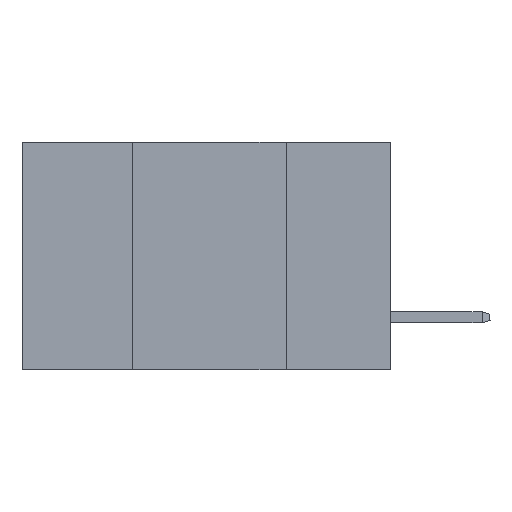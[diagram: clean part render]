
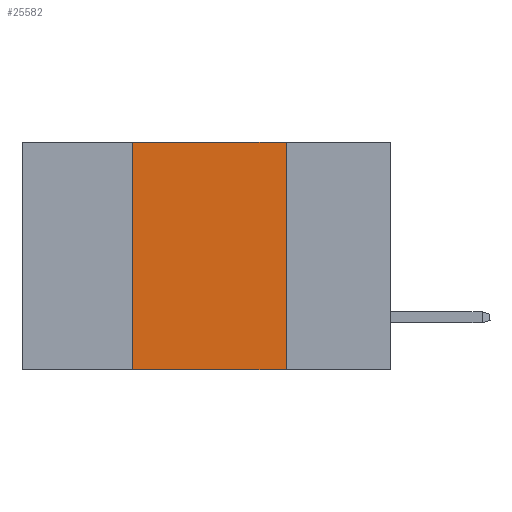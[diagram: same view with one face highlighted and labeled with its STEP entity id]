
A CAD part, left-side view. The second image highlights one B-rep face of the part: STEP entity #25582.
In plain terms, the highlighted planar face has unit normal (-1, 0, 0).
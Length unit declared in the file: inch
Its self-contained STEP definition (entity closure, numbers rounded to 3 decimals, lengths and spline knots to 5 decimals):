
#837 = AXIS2_PLACEMENT_3D ( 'NONE', #30326, #23139, #1492 ) ;
#848 = VECTOR ( 'NONE', #13029, 39.37008 ) ;
#1337 = FACE_OUTER_BOUND ( 'NONE', #26784, .T. ) ;
#1492 = DIRECTION ( 'NONE',  ( 0., 0., -1. ) ) ;
#1990 = DIRECTION ( 'NONE',  ( 0., -1., 0. ) ) ;
#3159 = LINE ( 'NONE', #29213, #7681 ) ;
#3954 = VECTOR ( 'NONE', #12092, 39.37008 ) ;
#4005 = EDGE_CURVE ( 'NONE', #14840, #10749, #11437, .T. ) ;
#5604 = LINE ( 'NONE', #9173, #28607 ) ;
#7681 = VECTOR ( 'NONE', #22342, 39.37008 ) ;
#8096 = CARTESIAN_POINT ( 'NONE',  ( 0., 0.17, -0.37 ) ) ;
#8244 = CARTESIAN_POINT ( 'NONE',  ( 0., 0.42, -0.37 ) ) ;
#9050 = EDGE_CURVE ( 'NONE', #12423, #14840, #3159, .T. ) ;
#9173 = CARTESIAN_POINT ( 'NONE',  ( 0., 0.6, -0.37 ) ) ;
#9866 = ORIENTED_EDGE ( 'NONE', *, *, #9050, .F. ) ;
#10749 = VERTEX_POINT ( 'NONE', #8096 ) ;
#11437 = LINE ( 'NONE', #12922, #848 ) ;
#12092 = DIRECTION ( 'NONE',  ( 0., 0., 1. ) ) ;
#12423 = VERTEX_POINT ( 'NONE', #16876 ) ;
#12580 = ORIENTED_EDGE ( 'NONE', *, *, #4005, .F. ) ;
#12769 = EDGE_CURVE ( 'NONE', #28000, #10749, #5604, .T. ) ;
#12922 = CARTESIAN_POINT ( 'NONE',  ( 0., 0.17, 0. ) ) ;
#13029 = DIRECTION ( 'NONE',  ( 0., 0., -1. ) ) ;
#14840 = VERTEX_POINT ( 'NONE', #27680 ) ;
#16876 = CARTESIAN_POINT ( 'NONE',  ( 0., 0.42, 0. ) ) ;
#16998 = ORIENTED_EDGE ( 'NONE', *, *, #17954, .F. ) ;
#17546 = ORIENTED_EDGE ( 'NONE', *, *, #12769, .T. ) ;
#17954 = EDGE_CURVE ( 'NONE', #28000, #12423, #22689, .T. ) ;
#22342 = DIRECTION ( 'NONE',  ( 0., -1., 0. ) ) ;
#22689 = LINE ( 'NONE', #28731, #3954 ) ;
#23139 = DIRECTION ( 'NONE',  ( 1., 0., 0. ) ) ;
#25535 = PLANE ( 'NONE',  #837 ) ;
#25582 = ADVANCED_FACE ( 'NONE', ( #1337 ), #25535, .F. ) ;
#26784 = EDGE_LOOP ( 'NONE', ( #12580, #9866, #16998, #17546 ) ) ;
#27680 = CARTESIAN_POINT ( 'NONE',  ( 0., 0.17, 0. ) ) ;
#28000 = VERTEX_POINT ( 'NONE', #8244 ) ;
#28607 = VECTOR ( 'NONE', #1990, 39.37008 ) ;
#28731 = CARTESIAN_POINT ( 'NONE',  ( 0., 0.42, 0. ) ) ;
#29213 = CARTESIAN_POINT ( 'NONE',  ( 0., 0.6, 0. ) ) ;
#30326 = CARTESIAN_POINT ( 'NONE',  ( 0., 0.6, 0. ) ) ;
